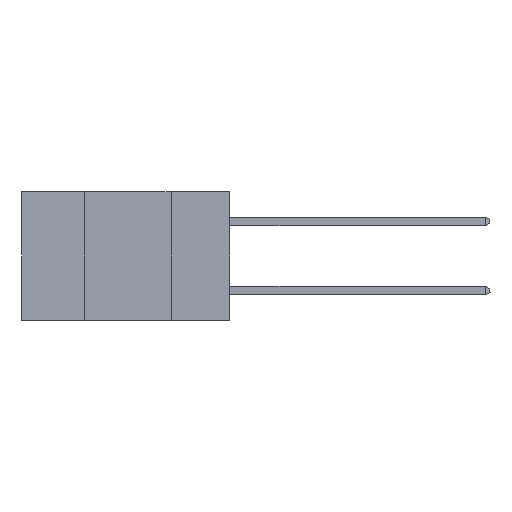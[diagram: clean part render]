
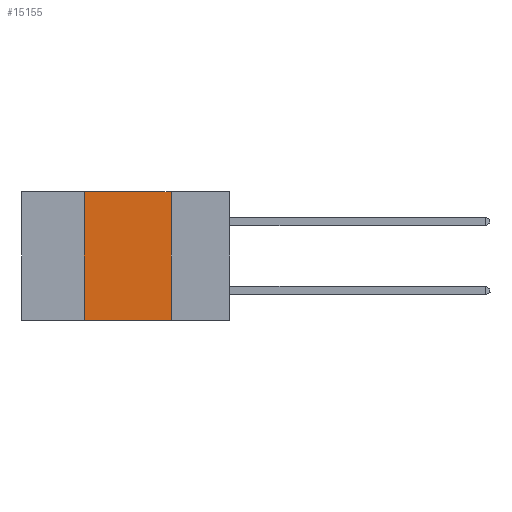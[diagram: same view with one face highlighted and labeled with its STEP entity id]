
A CAD part, left-side view. The second image highlights one B-rep face of the part: STEP entity #15155.
In plain terms, the highlighted planar face has unit normal (-1, 0, 0).
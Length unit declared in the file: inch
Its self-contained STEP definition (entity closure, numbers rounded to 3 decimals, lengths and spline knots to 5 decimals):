
#259 = ORIENTED_EDGE ( 'NONE', *, *, #14070, .F. ) ;
#545 = FACE_OUTER_BOUND ( 'NONE', #13210, .T. ) ;
#1672 = DIRECTION ( 'NONE',  ( 1., 0., 0. ) ) ;
#1744 = DIRECTION ( 'NONE',  ( 0., 0., -1. ) ) ;
#2384 = VECTOR ( 'NONE', #21432, 39.37008 ) ;
#2523 = LINE ( 'NONE', #4331, #15182 ) ;
#4331 = CARTESIAN_POINT ( 'NONE',  ( 0., 0.6, 0. ) ) ;
#4492 = EDGE_CURVE ( 'NONE', #7800, #16264, #2523, .T. ) ;
#5420 = CARTESIAN_POINT ( 'NONE',  ( 0., 0.17, -0.37 ) ) ;
#6412 = CARTESIAN_POINT ( 'NONE',  ( 0., 0.17, 0. ) ) ;
#6876 = VERTEX_POINT ( 'NONE', #5420 ) ;
#7800 = VERTEX_POINT ( 'NONE', #18975 ) ;
#8182 = DIRECTION ( 'NONE',  ( 0., 0., -1. ) ) ;
#8386 = CARTESIAN_POINT ( 'NONE',  ( 0., 0.42, 0. ) ) ;
#8551 = DIRECTION ( 'NONE',  ( 0., 0., 1. ) ) ;
#8871 = AXIS2_PLACEMENT_3D ( 'NONE', #19234, #1672, #1744 ) ;
#9672 = VECTOR ( 'NONE', #8182, 39.37008 ) ;
#10523 = EDGE_CURVE ( 'NONE', #14586, #6876, #16110, .T. ) ;
#12431 = VECTOR ( 'NONE', #8551, 39.37008 ) ;
#12953 = DIRECTION ( 'NONE',  ( 0., -1., 0. ) ) ;
#13210 = EDGE_LOOP ( 'NONE', ( #259, #21792, #21279, #14185 ) ) ;
#13250 = LINE ( 'NONE', #6412, #9672 ) ;
#13384 = CARTESIAN_POINT ( 'NONE',  ( 0., 0.42, -0.37 ) ) ;
#14070 = EDGE_CURVE ( 'NONE', #16264, #6876, #13250, .T. ) ;
#14094 = LINE ( 'NONE', #8386, #12431 ) ;
#14185 = ORIENTED_EDGE ( 'NONE', *, *, #10523, .T. ) ;
#14290 = CARTESIAN_POINT ( 'NONE',  ( 0., 0.6, -0.37 ) ) ;
#14586 = VERTEX_POINT ( 'NONE', #13384 ) ;
#15155 = ADVANCED_FACE ( 'NONE', ( #545 ), #19380, .F. ) ;
#15182 = VECTOR ( 'NONE', #12953, 39.37008 ) ;
#16110 = LINE ( 'NONE', #14290, #2384 ) ;
#16264 = VERTEX_POINT ( 'NONE', #16297 ) ;
#16297 = CARTESIAN_POINT ( 'NONE',  ( 0., 0.17, 0. ) ) ;
#17588 = EDGE_CURVE ( 'NONE', #14586, #7800, #14094, .T. ) ;
#18975 = CARTESIAN_POINT ( 'NONE',  ( 0., 0.42, 0. ) ) ;
#19234 = CARTESIAN_POINT ( 'NONE',  ( 0., 0.6, 0. ) ) ;
#19380 = PLANE ( 'NONE',  #8871 ) ;
#21279 = ORIENTED_EDGE ( 'NONE', *, *, #17588, .F. ) ;
#21432 = DIRECTION ( 'NONE',  ( 0., -1., 0. ) ) ;
#21792 = ORIENTED_EDGE ( 'NONE', *, *, #4492, .F. ) ;
